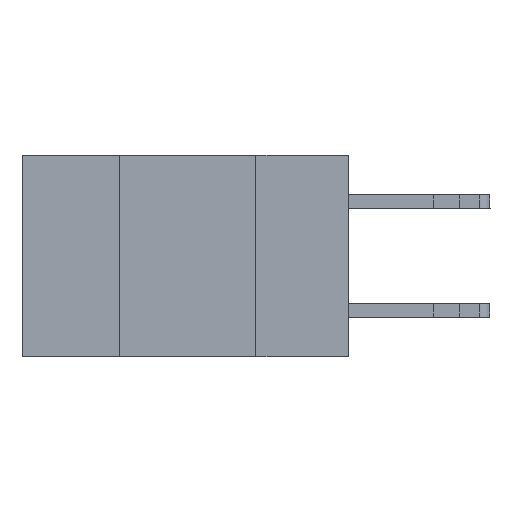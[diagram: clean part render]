
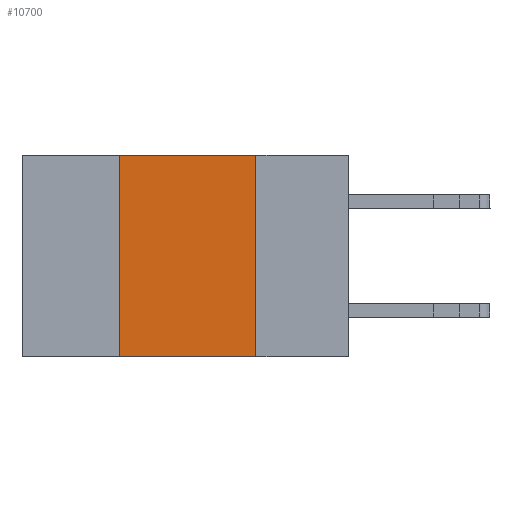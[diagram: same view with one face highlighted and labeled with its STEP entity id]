
A CAD part, left-side view. The second image highlights one B-rep face of the part: STEP entity #10700.
In plain terms, the highlighted planar face has unit normal (-1, 0, 0).
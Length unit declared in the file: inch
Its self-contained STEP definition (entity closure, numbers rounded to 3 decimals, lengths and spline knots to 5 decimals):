
#112 = ORIENTED_EDGE ( 'NONE', *, *, #11973, .F. ) ;
#772 = DIRECTION ( 'NONE',  ( 1., 0., 0. ) ) ;
#1015 = CARTESIAN_POINT ( 'NONE',  ( 0., 0.17, 0. ) ) ;
#1736 = CARTESIAN_POINT ( 'NONE',  ( 0., 0.6, 0. ) ) ;
#2014 = VERTEX_POINT ( 'NONE', #5829 ) ;
#2466 = AXIS2_PLACEMENT_3D ( 'NONE', #1736, #772, #14678 ) ;
#2703 = VERTEX_POINT ( 'NONE', #12673 ) ;
#3118 = VERTEX_POINT ( 'NONE', #1015 ) ;
#3663 = EDGE_LOOP ( 'NONE', ( #3969, #112, #4333, #13308 ) ) ;
#3969 = ORIENTED_EDGE ( 'NONE', *, *, #14411, .F. ) ;
#4167 = LINE ( 'NONE', #6344, #9227 ) ;
#4245 = LINE ( 'NONE', #6750, #5154 ) ;
#4333 = ORIENTED_EDGE ( 'NONE', *, *, #11798, .F. ) ;
#5139 = CARTESIAN_POINT ( 'NONE',  ( 0., 0.17, -0.37 ) ) ;
#5154 = VECTOR ( 'NONE', #10041, 39.37008 ) ;
#5437 = VECTOR ( 'NONE', #14448, 39.37008 ) ;
#5564 = LINE ( 'NONE', #9844, #5437 ) ;
#5829 = CARTESIAN_POINT ( 'NONE',  ( 0., 0.42, -0.37 ) ) ;
#6344 = CARTESIAN_POINT ( 'NONE',  ( 0., 0.6, -0.37 ) ) ;
#6750 = CARTESIAN_POINT ( 'NONE',  ( 0., 0.6, 0. ) ) ;
#7659 = DIRECTION ( 'NONE',  ( 0., -1., 0. ) ) ;
#8624 = DIRECTION ( 'NONE',  ( 0., 0., -1. ) ) ;
#8786 = FACE_OUTER_BOUND ( 'NONE', #3663, .T. ) ;
#9062 = VECTOR ( 'NONE', #8624, 39.37008 ) ;
#9227 = VECTOR ( 'NONE', #7659, 39.37008 ) ;
#9663 = LINE ( 'NONE', #5139, #9062 ) ;
#9844 = CARTESIAN_POINT ( 'NONE',  ( 0., 0.42, -0.37 ) ) ;
#9908 = PLANE ( 'NONE',  #2466 ) ;
#10041 = DIRECTION ( 'NONE',  ( 0., -1., 0. ) ) ;
#10700 = ADVANCED_FACE ( 'NONE', ( #8786 ), #9908, .F. ) ;
#11018 = EDGE_CURVE ( 'NONE', #2014, #2703, #4167, .T. ) ;
#11798 = EDGE_CURVE ( 'NONE', #2014, #12777, #5564, .T. ) ;
#11973 = EDGE_CURVE ( 'NONE', #12777, #3118, #4245, .T. ) ;
#12673 = CARTESIAN_POINT ( 'NONE',  ( 0., 0.17, -0.37 ) ) ;
#12777 = VERTEX_POINT ( 'NONE', #12910 ) ;
#12910 = CARTESIAN_POINT ( 'NONE',  ( 0., 0.42, 0. ) ) ;
#13308 = ORIENTED_EDGE ( 'NONE', *, *, #11018, .T. ) ;
#14411 = EDGE_CURVE ( 'NONE', #3118, #2703, #9663, .T. ) ;
#14448 = DIRECTION ( 'NONE',  ( 0., 0., 1. ) ) ;
#14678 = DIRECTION ( 'NONE',  ( 0., 0., -1. ) ) ;
